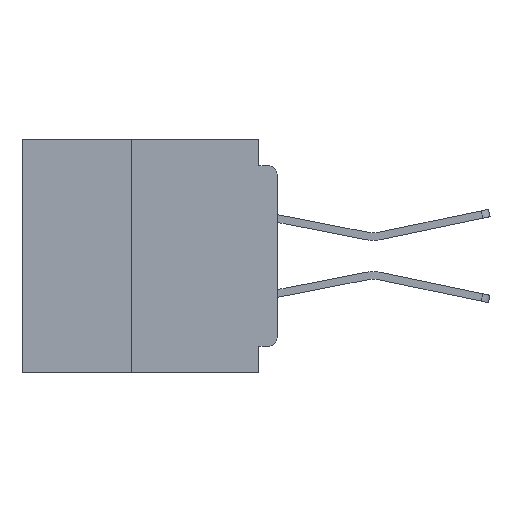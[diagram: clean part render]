
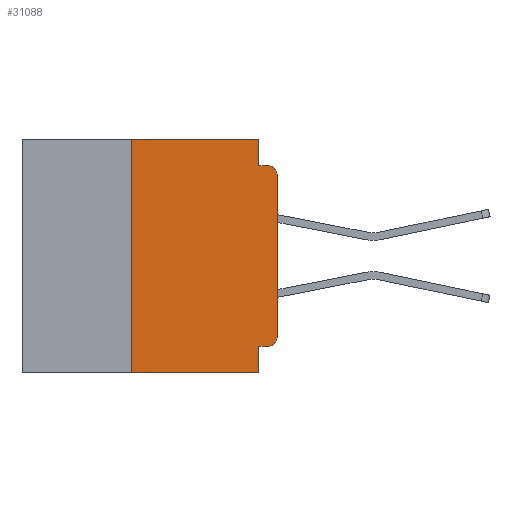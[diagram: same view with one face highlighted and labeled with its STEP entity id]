
A CAD part, left-side view. The second image highlights one B-rep face of the part: STEP entity #31088.
In plain terms, the highlighted planar face has unit normal (-1, 0, 0).
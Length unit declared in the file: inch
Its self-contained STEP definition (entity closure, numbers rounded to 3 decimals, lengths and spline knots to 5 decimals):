
#119 = VECTOR ( 'NONE', #5028, 39.37008 ) ;
#447 = CARTESIAN_POINT ( 'NONE',  ( 0., 0., -0.355 ) ) ;
#798 = CARTESIAN_POINT ( 'NONE',  ( 0., 0.031, -0.4 ) ) ;
#1210 = LINE ( 'NONE', #29678, #119 ) ;
#1334 = LINE ( 'NONE', #44426, #19140 ) ;
#1469 = ORIENTED_EDGE ( 'NONE', *, *, #28268, .F. ) ;
#1946 = DIRECTION ( 'NONE',  ( 0., -1., 0. ) ) ;
#3675 = ORIENTED_EDGE ( 'NONE', *, *, #22564, .T. ) ;
#3679 = VECTOR ( 'NONE', #19548, 39.37008 ) ;
#4639 = CARTESIAN_POINT ( 'NONE',  ( 0., 0.015, -0.06 ) ) ;
#4777 = VECTOR ( 'NONE', #18186, 39.37008 ) ;
#5028 = DIRECTION ( 'NONE',  ( 0., -1., 0. ) ) ;
#5446 = CARTESIAN_POINT ( 'NONE',  ( 0., 0.437, 0. ) ) ;
#6232 = DIRECTION ( 'NONE',  ( 0., -1., 0. ) ) ;
#6732 = CARTESIAN_POINT ( 'NONE',  ( 0., 0.015, -0.34 ) ) ;
#7734 = EDGE_CURVE ( 'NONE', #33279, #35079, #1210, .T. ) ;
#7944 = LINE ( 'NONE', #15443, #26681 ) ;
#8222 = ORIENTED_EDGE ( 'NONE', *, *, #10304, .F. ) ;
#8240 = DIRECTION ( 'NONE',  ( 0., 0., -1. ) ) ;
#9294 = DIRECTION ( 'NONE',  ( 0., 0., 1. ) ) ;
#9657 = CARTESIAN_POINT ( 'NONE',  ( 0., 0.437, -0.4 ) ) ;
#9661 = ORIENTED_EDGE ( 'NONE', *, *, #12425, .F. ) ;
#10242 = VECTOR ( 'NONE', #1946, 39.37008 ) ;
#10304 = EDGE_CURVE ( 'NONE', #35079, #25775, #13154, .T. ) ;
#10323 = DIRECTION ( 'NONE',  ( 0., 0., -1. ) ) ;
#10519 = CARTESIAN_POINT ( 'NONE',  ( 0., 0.25, 0. ) ) ;
#11151 = VERTEX_POINT ( 'NONE', #24346 ) ;
#11339 = EDGE_CURVE ( 'NONE', #16142, #25153, #44856, .T. ) ;
#11926 = EDGE_CURVE ( 'NONE', #25775, #43378, #19644, .T. ) ;
#12419 = CARTESIAN_POINT ( 'NONE',  ( 0., 0.031, 0. ) ) ;
#12425 = EDGE_CURVE ( 'NONE', #11151, #33279, #7944, .T. ) ;
#13154 = LINE ( 'NONE', #12419, #3679 ) ;
#13946 = VERTEX_POINT ( 'NONE', #26931 ) ;
#15443 = CARTESIAN_POINT ( 'NONE',  ( 0., 0.25, -0.4 ) ) ;
#16142 = VERTEX_POINT ( 'NONE', #40140 ) ;
#16175 = DIRECTION ( 'NONE',  ( 0., 0., -1. ) ) ;
#18186 = DIRECTION ( 'NONE',  ( 0., 1., 0. ) ) ;
#18543 = DIRECTION ( 'NONE',  ( 0., 0., -1. ) ) ;
#19140 = VECTOR ( 'NONE', #9294, 39.37008 ) ;
#19548 = DIRECTION ( 'NONE',  ( 0., 0., -1. ) ) ;
#19644 = LINE ( 'NONE', #44104, #10242 ) ;
#20402 = ORIENTED_EDGE ( 'NONE', *, *, #43703, .T. ) ;
#22564 = EDGE_CURVE ( 'NONE', #11151, #25153, #39944, .T. ) ;
#23603 = LINE ( 'NONE', #447, #4777 ) ;
#24346 = CARTESIAN_POINT ( 'NONE',  ( 0., 0.25, -0.4 ) ) ;
#24705 = CIRCLE ( 'NONE', #41746, 0.015 ) ;
#25153 = VERTEX_POINT ( 'NONE', #35179 ) ;
#25775 = VERTEX_POINT ( 'NONE', #34979 ) ;
#26248 = VECTOR ( 'NONE', #18543, 39.37008 ) ;
#26681 = VECTOR ( 'NONE', #36389, 39.37008 ) ;
#26931 = CARTESIAN_POINT ( 'NONE',  ( 0., 0., -0.34 ) ) ;
#28268 = EDGE_CURVE ( 'NONE', #44802, #16142, #23603, .T. ) ;
#28905 = VERTEX_POINT ( 'NONE', #32001 ) ;
#29309 = DIRECTION ( 'NONE',  ( -1., 0., 0. ) ) ;
#29678 = CARTESIAN_POINT ( 'NONE',  ( 0., 0.437, 0. ) ) ;
#30611 = VECTOR ( 'NONE', #6232, 39.37008 ) ;
#30815 = AXIS2_PLACEMENT_3D ( 'NONE', #5446, #37118, #16175 ) ;
#31088 = ADVANCED_FACE ( 'NONE', ( #34253 ), #44028, .F. ) ;
#31331 = DIRECTION ( 'NONE',  ( -1., 0., 0. ) ) ;
#32001 = CARTESIAN_POINT ( 'NONE',  ( 0., 0., -0.06 ) ) ;
#32784 = ORIENTED_EDGE ( 'NONE', *, *, #33829, .T. ) ;
#33279 = VERTEX_POINT ( 'NONE', #10519 ) ;
#33291 = EDGE_LOOP ( 'NONE', ( #35483, #20402, #40776, #8222, #42442, #9661, #3675, #34266, #1469, #32784 ) ) ;
#33829 = EDGE_CURVE ( 'NONE', #44802, #13946, #24705, .T. ) ;
#34253 = FACE_OUTER_BOUND ( 'NONE', #33291, .T. ) ;
#34266 = ORIENTED_EDGE ( 'NONE', *, *, #11339, .F. ) ;
#34979 = CARTESIAN_POINT ( 'NONE',  ( 0., 0.031, -0.045 ) ) ;
#35079 = VERTEX_POINT ( 'NONE', #39720 ) ;
#35179 = CARTESIAN_POINT ( 'NONE',  ( 0., 0.031, -0.4 ) ) ;
#35483 = ORIENTED_EDGE ( 'NONE', *, *, #39110, .T. ) ;
#36389 = DIRECTION ( 'NONE',  ( 0., 0., 1. ) ) ;
#37118 = DIRECTION ( 'NONE',  ( 1., 0., 0. ) ) ;
#39110 = EDGE_CURVE ( 'NONE', #13946, #28905, #1334, .T. ) ;
#39720 = CARTESIAN_POINT ( 'NONE',  ( 0., 0.031, 0. ) ) ;
#39763 = AXIS2_PLACEMENT_3D ( 'NONE', #4639, #29309, #8240 ) ;
#39944 = LINE ( 'NONE', #9657, #30611 ) ;
#40140 = CARTESIAN_POINT ( 'NONE',  ( 0., 0.031, -0.355 ) ) ;
#40776 = ORIENTED_EDGE ( 'NONE', *, *, #11926, .F. ) ;
#41746 = AXIS2_PLACEMENT_3D ( 'NONE', #6732, #31331, #10323 ) ;
#42442 = ORIENTED_EDGE ( 'NONE', *, *, #7734, .F. ) ;
#43288 = CIRCLE ( 'NONE', #39763, 0.015 ) ;
#43378 = VERTEX_POINT ( 'NONE', #45091 ) ;
#43703 = EDGE_CURVE ( 'NONE', #28905, #43378, #43288, .T. ) ;
#44028 = PLANE ( 'NONE',  #30815 ) ;
#44104 = CARTESIAN_POINT ( 'NONE',  ( 0., 0., -0.045 ) ) ;
#44197 = CARTESIAN_POINT ( 'NONE',  ( 0., 0.015, -0.355 ) ) ;
#44426 = CARTESIAN_POINT ( 'NONE',  ( 0., 0., 0. ) ) ;
#44802 = VERTEX_POINT ( 'NONE', #44197 ) ;
#44856 = LINE ( 'NONE', #798, #26248 ) ;
#45091 = CARTESIAN_POINT ( 'NONE',  ( 0., 0.015, -0.045 ) ) ;
